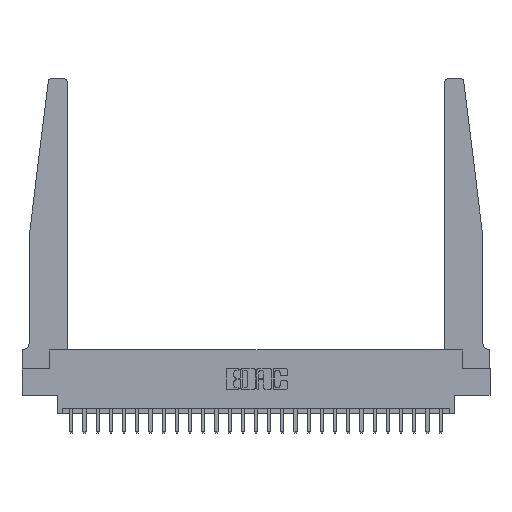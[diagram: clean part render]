
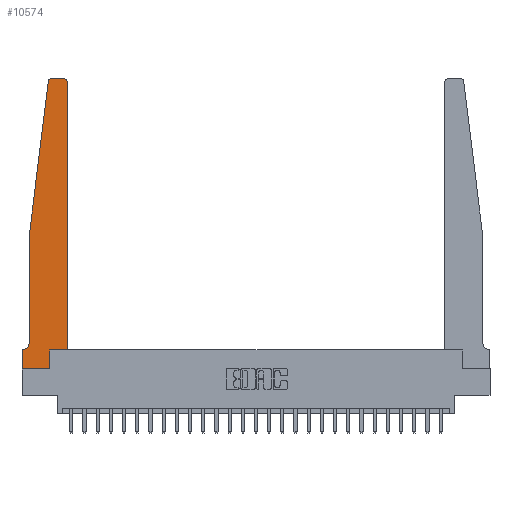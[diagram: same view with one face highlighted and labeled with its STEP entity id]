
A CAD part, top view. The second image highlights one B-rep face of the part: STEP entity #10574.
In plain terms, the highlighted planar face has unit normal (0, 0, 1).
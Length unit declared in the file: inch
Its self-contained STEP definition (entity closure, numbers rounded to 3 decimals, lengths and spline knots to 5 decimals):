
#700 = CARTESIAN_POINT ( 'NONE',  ( 0.27653, 2.72, 0.37 ) ) ;
#831 = DIRECTION ( 'NONE',  ( 1., 0., 0. ) ) ;
#1111 = CARTESIAN_POINT ( 'NONE',  ( 0.27653, 2.75, 0.37 ) ) ;
#1824 = DIRECTION ( 'NONE',  ( -1., 0., 0. ) ) ;
#2479 = VECTOR ( 'NONE', #22904, 39.37008 ) ;
#2626 = CARTESIAN_POINT ( 'NONE',  ( 0.015, 0.1875, 0.37 ) ) ;
#2653 = EDGE_CURVE ( 'NONE', #7727, #13322, #11520, .T. ) ;
#2673 = ORIENTED_EDGE ( 'NONE', *, *, #25594, .T. ) ;
#2801 = DIRECTION ( 'NONE',  ( 1., 0., 0. ) ) ;
#2847 = VECTOR ( 'NONE', #23021, 39.37008 ) ;
#3313 = LINE ( 'NONE', #17688, #17909 ) ;
#3417 = EDGE_CURVE ( 'NONE', #4872, #25155, #19518, .T. ) ;
#3418 = ORIENTED_EDGE ( 'NONE', *, *, #14366, .T. ) ;
#3901 = ORIENTED_EDGE ( 'NONE', *, *, #24540, .T. ) ;
#4220 = FACE_OUTER_BOUND ( 'NONE', #23214, .T. ) ;
#4554 = CARTESIAN_POINT ( 'NONE',  ( 0.24675, 2.72367, 0.37 ) ) ;
#4555 = VECTOR ( 'NONE', #11216, 39.37008 ) ;
#4591 = DIRECTION ( 'NONE',  ( 1., 0., 0. ) ) ;
#4767 = VERTEX_POINT ( 'NONE', #5460 ) ;
#4872 = VERTEX_POINT ( 'NONE', #14001 ) ;
#5162 = DIRECTION ( 'NONE',  ( 1., 0., 0. ) ) ;
#5200 = CARTESIAN_POINT ( 'NONE',  ( 0.2605, 0.18, 0.37 ) ) ;
#5348 = VECTOR ( 'NONE', #16105, 39.37008 ) ;
#5460 = CARTESIAN_POINT ( 'NONE',  ( 0.065, 1.25, 0.37 ) ) ;
#6305 = VECTOR ( 'NONE', #20484, 39.37008 ) ;
#6353 = ORIENTED_EDGE ( 'NONE', *, *, #22863, .T. ) ;
#6450 = DIRECTION ( 'NONE',  ( -1., 0., 0. ) ) ;
#6474 = DIRECTION ( 'NONE',  ( 0., 0., -1. ) ) ;
#6481 = CARTESIAN_POINT ( 'NONE',  ( 0.015, 0.2375, 0.37 ) ) ;
#6661 = AXIS2_PLACEMENT_3D ( 'NONE', #8330, #16524, #4591 ) ;
#6834 = ORIENTED_EDGE ( 'NONE', *, *, #20592, .T. ) ;
#6962 = LINE ( 'NONE', #18513, #6305 ) ;
#7149 = VERTEX_POINT ( 'NONE', #18553 ) ;
#7214 = EDGE_CURVE ( 'NONE', #9377, #7149, #7238, .T. ) ;
#7238 = LINE ( 'NONE', #8988, #13113 ) ;
#7425 = VERTEX_POINT ( 'NONE', #11554 ) ;
#7544 = EDGE_CURVE ( 'NONE', #25155, #25312, #16197, .T. ) ;
#7727 = VERTEX_POINT ( 'NONE', #12571 ) ;
#8330 = CARTESIAN_POINT ( 'NONE',  ( 0., 0.1875, 0.37 ) ) ;
#8988 = CARTESIAN_POINT ( 'NONE',  ( 0., 0., 0.37 ) ) ;
#9144 = EDGE_CURVE ( 'NONE', #13322, #9377, #3313, .T. ) ;
#9377 = VERTEX_POINT ( 'NONE', #24244 ) ;
#9648 = VECTOR ( 'NONE', #5162, 39.37008 ) ;
#9767 = CARTESIAN_POINT ( 'NONE',  ( 0.395, 2.75, 0.37 ) ) ;
#10030 = AXIS2_PLACEMENT_3D ( 'NONE', #6481, #6474, #6450 ) ;
#10305 = VECTOR ( 'NONE', #13905, 39.37008 ) ;
#10574 = ADVANCED_FACE ( 'NONE', ( #4220 ), #12261, .T. ) ;
#11102 = VERTEX_POINT ( 'NONE', #4554 ) ;
#11124 = CARTESIAN_POINT ( 'NONE',  ( 0.425, 0.18, 0.37 ) ) ;
#11145 = CARTESIAN_POINT ( 'NONE',  ( 0., 0., 0.37 ) ) ;
#11216 = DIRECTION ( 'NONE',  ( 0., 1., 0. ) ) ;
#11520 = CIRCLE ( 'NONE', #10030, 0.05 ) ;
#11554 = CARTESIAN_POINT ( 'NONE',  ( 0.2605, 0., 0.37 ) ) ;
#12239 = CIRCLE ( 'NONE', #15906, 0.03 ) ;
#12261 = PLANE ( 'NONE',  #6661 ) ;
#12571 = CARTESIAN_POINT ( 'NONE',  ( 0.065, 0.2375, 0.37 ) ) ;
#12888 = DIRECTION ( 'NONE',  ( 0., 0., 1. ) ) ;
#13113 = VECTOR ( 'NONE', #22642, 39.37008 ) ;
#13322 = VERTEX_POINT ( 'NONE', #2626 ) ;
#13454 = CIRCLE ( 'NONE', #22971, 0.03 ) ;
#13905 = DIRECTION ( 'NONE',  ( 0., 1., 0. ) ) ;
#14001 = CARTESIAN_POINT ( 'NONE',  ( 0.2605, 0.18, 0.37 ) ) ;
#14004 = EDGE_CURVE ( 'NONE', #14733, #17021, #18703, .T. ) ;
#14366 = EDGE_CURVE ( 'NONE', #11102, #4767, #15927, .T. ) ;
#14706 = EDGE_CURVE ( 'NONE', #7149, #7425, #22925, .T. ) ;
#14733 = VERTEX_POINT ( 'NONE', #9767 ) ;
#14757 = DIRECTION ( 'NONE',  ( 0., 0., 1. ) ) ;
#15721 = CARTESIAN_POINT ( 'NONE',  ( 0.425, 2.72, 0.37 ) ) ;
#15906 = AXIS2_PLACEMENT_3D ( 'NONE', #700, #14757, #2801 ) ;
#15927 = LINE ( 'NONE', #21892, #5348 ) ;
#16105 = DIRECTION ( 'NONE',  ( -0.122, -0.992, 0. ) ) ;
#16197 = LINE ( 'NONE', #23631, #10305 ) ;
#16524 = DIRECTION ( 'NONE',  ( 0., 0., 1. ) ) ;
#17021 = VERTEX_POINT ( 'NONE', #1111 ) ;
#17063 = CARTESIAN_POINT ( 'NONE',  ( 0.425, 0.18, 0.37 ) ) ;
#17330 = ORIENTED_EDGE ( 'NONE', *, *, #2653, .T. ) ;
#17688 = CARTESIAN_POINT ( 'NONE',  ( 0.065, 0.1875, 0.37 ) ) ;
#17909 = VECTOR ( 'NONE', #1824, 39.37008 ) ;
#18513 = CARTESIAN_POINT ( 'NONE',  ( 0.065, 1.25, 0.37 ) ) ;
#18553 = CARTESIAN_POINT ( 'NONE',  ( 0., 0., 0.37 ) ) ;
#18703 = LINE ( 'NONE', #21067, #2847 ) ;
#19518 = LINE ( 'NONE', #17063, #9648 ) ;
#20272 = ORIENTED_EDGE ( 'NONE', *, *, #3417, .T. ) ;
#20382 = LINE ( 'NONE', #5200, #4555 ) ;
#20484 = DIRECTION ( 'NONE',  ( 0., -1., 0. ) ) ;
#20592 = EDGE_CURVE ( 'NONE', #7425, #4872, #20382, .T. ) ;
#21067 = CARTESIAN_POINT ( 'NONE',  ( 0.25, 2.75, 0.37 ) ) ;
#21795 = ORIENTED_EDGE ( 'NONE', *, *, #7544, .T. ) ;
#21892 = CARTESIAN_POINT ( 'NONE',  ( 0.065, 1.25, 0.37 ) ) ;
#22296 = ORIENTED_EDGE ( 'NONE', *, *, #7214, .T. ) ;
#22642 = DIRECTION ( 'NONE',  ( 0., -1., 0. ) ) ;
#22747 = ORIENTED_EDGE ( 'NONE', *, *, #14004, .T. ) ;
#22863 = EDGE_CURVE ( 'NONE', #17021, #11102, #12239, .T. ) ;
#22904 = DIRECTION ( 'NONE',  ( 1., 0., 0. ) ) ;
#22925 = LINE ( 'NONE', #11145, #2479 ) ;
#22971 = AXIS2_PLACEMENT_3D ( 'NONE', #24615, #12888, #831 ) ;
#23021 = DIRECTION ( 'NONE',  ( -1., 0., 0. ) ) ;
#23214 = EDGE_LOOP ( 'NONE', ( #22747, #6353, #3418, #2673, #17330, #25089, #22296, #24579, #6834, #20272, #21795, #3901 ) ) ;
#23631 = CARTESIAN_POINT ( 'NONE',  ( 0.425, 0.18, 0.37 ) ) ;
#24244 = CARTESIAN_POINT ( 'NONE',  ( 0., 0.1875, 0.37 ) ) ;
#24540 = EDGE_CURVE ( 'NONE', #25312, #14733, #13454, .T. ) ;
#24579 = ORIENTED_EDGE ( 'NONE', *, *, #14706, .T. ) ;
#24615 = CARTESIAN_POINT ( 'NONE',  ( 0.395, 2.72, 0.37 ) ) ;
#25089 = ORIENTED_EDGE ( 'NONE', *, *, #9144, .T. ) ;
#25155 = VERTEX_POINT ( 'NONE', #11124 ) ;
#25312 = VERTEX_POINT ( 'NONE', #15721 ) ;
#25594 = EDGE_CURVE ( 'NONE', #4767, #7727, #6962, .T. ) ;
